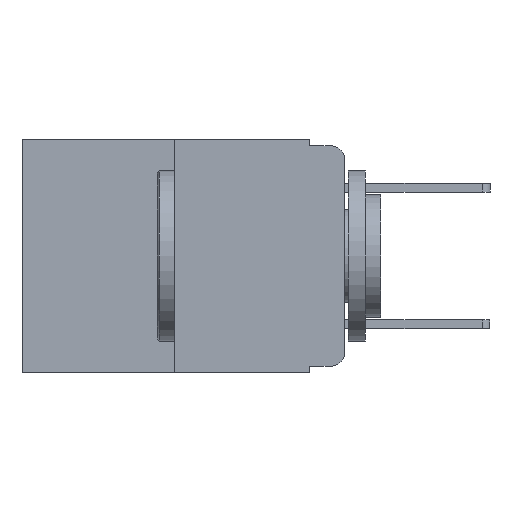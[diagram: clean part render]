
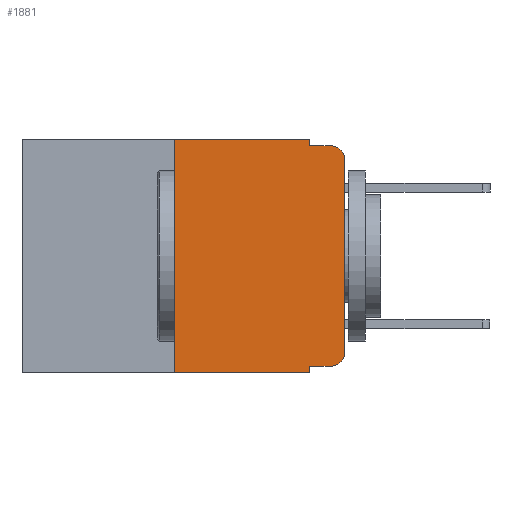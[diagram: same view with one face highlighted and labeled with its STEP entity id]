
A CAD part, left-side view. The second image highlights one B-rep face of the part: STEP entity #1881.
In plain terms, the highlighted planar face has unit normal (-1, 0, 0).
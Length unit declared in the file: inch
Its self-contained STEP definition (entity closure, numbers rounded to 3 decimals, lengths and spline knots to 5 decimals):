
#32 = VERTEX_POINT ( 'NONE', #5158 ) ;
#38 = CARTESIAN_POINT ( 'NONE',  ( 0., 0., -0.03 ) ) ;
#203 = EDGE_CURVE ( 'NONE', #1084, #32, #5326, .T. ) ;
#222 = ORIENTED_EDGE ( 'NONE', *, *, #20302, .T. ) ;
#477 = VECTOR ( 'NONE', #18074, 39.37008 ) ;
#578 = EDGE_CURVE ( 'NONE', #7838, #6584, #17220, .T. ) ;
#1083 = VERTEX_POINT ( 'NONE', #1965 ) ;
#1084 = VERTEX_POINT ( 'NONE', #23233 ) ;
#1786 = ORIENTED_EDGE ( 'NONE', *, *, #15106, .F. ) ;
#1881 = ADVANCED_FACE ( 'NONE', ( #24767 ), #8391, .F. ) ;
#1965 = CARTESIAN_POINT ( 'NONE',  ( 0., 0.051, -0.333 ) ) ;
#3151 = DIRECTION ( 'NONE',  ( -1., 0., 0. ) ) ;
#3761 = VERTEX_POINT ( 'NONE', #13410 ) ;
#3836 = CARTESIAN_POINT ( 'NONE',  ( 0., 0.051, 0. ) ) ;
#3948 = EDGE_CURVE ( 'NONE', #3761, #16313, #25304, .T. ) ;
#3993 = ORIENTED_EDGE ( 'NONE', *, *, #7341, .F. ) ;
#4042 = VECTOR ( 'NONE', #17843, 39.37008 ) ;
#4272 = CIRCLE ( 'NONE', #21971, 0.02 ) ;
#4856 = VECTOR ( 'NONE', #9632, 39.37008 ) ;
#4881 = ORIENTED_EDGE ( 'NONE', *, *, #10734, .T. ) ;
#4943 = DIRECTION ( 'NONE',  ( 0., 0., 1. ) ) ;
#5158 = CARTESIAN_POINT ( 'NONE',  ( 0., 0.051, 0. ) ) ;
#5326 = LINE ( 'NONE', #5982, #25729 ) ;
#5420 = EDGE_CURVE ( 'NONE', #16352, #24454, #21379, .T. ) ;
#5564 = ORIENTED_EDGE ( 'NONE', *, *, #3948, .T. ) ;
#5982 = CARTESIAN_POINT ( 'NONE',  ( 0., 0.473, 0. ) ) ;
#6281 = VECTOR ( 'NONE', #4943, 39.37008 ) ;
#6502 = EDGE_CURVE ( 'NONE', #32, #7838, #22802, .T. ) ;
#6584 = VERTEX_POINT ( 'NONE', #23569 ) ;
#7341 = EDGE_CURVE ( 'NONE', #1083, #16313, #19396, .T. ) ;
#7838 = VERTEX_POINT ( 'NONE', #24963 ) ;
#8124 = DIRECTION ( 'NONE',  ( 0., -1., 0. ) ) ;
#8391 = PLANE ( 'NONE',  #11916 ) ;
#8886 = CARTESIAN_POINT ( 'NONE',  ( 0., 0., 0. ) ) ;
#9097 = CARTESIAN_POINT ( 'NONE',  ( 0., 0.473, 0. ) ) ;
#9177 = DIRECTION ( 'NONE',  ( 1., 0., 0. ) ) ;
#9498 = CARTESIAN_POINT ( 'NONE',  ( 0., 0.051, 0. ) ) ;
#9632 = DIRECTION ( 'NONE',  ( 0., -1., 0. ) ) ;
#10734 = EDGE_CURVE ( 'NONE', #24454, #6584, #20980, .T. ) ;
#10807 = VECTOR ( 'NONE', #13943, 39.37008 ) ;
#10995 = CARTESIAN_POINT ( 'NONE',  ( 0., 0.02, -0.313 ) ) ;
#11696 = LINE ( 'NONE', #18957, #6281 ) ;
#11853 = LINE ( 'NONE', #17999, #477 ) ;
#11916 = AXIS2_PLACEMENT_3D ( 'NONE', #9097, #9177, #13245 ) ;
#11947 = VECTOR ( 'NONE', #8124, 39.37008 ) ;
#12475 = ORIENTED_EDGE ( 'NONE', *, *, #203, .F. ) ;
#12910 = CARTESIAN_POINT ( 'NONE',  ( 0., 0., -0.313 ) ) ;
#13019 = DIRECTION ( 'NONE',  ( 0., 0., -1. ) ) ;
#13245 = DIRECTION ( 'NONE',  ( 0., 0., -1. ) ) ;
#13410 = CARTESIAN_POINT ( 'NONE',  ( 0., 0.25, -0.343 ) ) ;
#13437 = CARTESIAN_POINT ( 'NONE',  ( 0., 0.473, -0.343 ) ) ;
#13943 = DIRECTION ( 'NONE',  ( 0., 0., 1. ) ) ;
#14121 = DIRECTION ( 'NONE',  ( 0., -1., 0. ) ) ;
#15106 = EDGE_CURVE ( 'NONE', #3761, #1084, #11696, .T. ) ;
#15167 = CARTESIAN_POINT ( 'NONE',  ( 0., 0.02, -0.03 ) ) ;
#15232 = AXIS2_PLACEMENT_3D ( 'NONE', #15167, #3151, #17163 ) ;
#15510 = DIRECTION ( 'NONE',  ( 0., 0., -1. ) ) ;
#16313 = VERTEX_POINT ( 'NONE', #24559 ) ;
#16352 = VERTEX_POINT ( 'NONE', #12910 ) ;
#17163 = DIRECTION ( 'NONE',  ( 0., 0., -1. ) ) ;
#17220 = LINE ( 'NONE', #25060, #11947 ) ;
#17581 = VECTOR ( 'NONE', #15510, 39.37008 ) ;
#17843 = DIRECTION ( 'NONE',  ( 0., 0., -1. ) ) ;
#17999 = CARTESIAN_POINT ( 'NONE',  ( 0., 0.051, -0.333 ) ) ;
#18074 = DIRECTION ( 'NONE',  ( 0., -1., 0. ) ) ;
#18192 = VERTEX_POINT ( 'NONE', #20888 ) ;
#18957 = CARTESIAN_POINT ( 'NONE',  ( 0., 0.25, 0. ) ) ;
#19396 = LINE ( 'NONE', #3836, #4042 ) ;
#20194 = EDGE_LOOP ( 'NONE', ( #25609, #4881, #23271, #24431, #12475, #1786, #5564, #3993, #20554, #222 ) ) ;
#20302 = EDGE_CURVE ( 'NONE', #18192, #16352, #4272, .T. ) ;
#20554 = ORIENTED_EDGE ( 'NONE', *, *, #23187, .T. ) ;
#20888 = CARTESIAN_POINT ( 'NONE',  ( 0., 0.02, -0.333 ) ) ;
#20980 = CIRCLE ( 'NONE', #15232, 0.02 ) ;
#21379 = LINE ( 'NONE', #8886, #10807 ) ;
#21971 = AXIS2_PLACEMENT_3D ( 'NONE', #10995, #24761, #13019 ) ;
#22802 = LINE ( 'NONE', #9498, #17581 ) ;
#23187 = EDGE_CURVE ( 'NONE', #1083, #18192, #11853, .T. ) ;
#23233 = CARTESIAN_POINT ( 'NONE',  ( 0., 0.25, 0. ) ) ;
#23271 = ORIENTED_EDGE ( 'NONE', *, *, #578, .F. ) ;
#23569 = CARTESIAN_POINT ( 'NONE',  ( 0., 0.02, -0.01 ) ) ;
#24431 = ORIENTED_EDGE ( 'NONE', *, *, #6502, .F. ) ;
#24454 = VERTEX_POINT ( 'NONE', #38 ) ;
#24559 = CARTESIAN_POINT ( 'NONE',  ( 0., 0.051, -0.343 ) ) ;
#24761 = DIRECTION ( 'NONE',  ( -1., 0., 0. ) ) ;
#24767 = FACE_OUTER_BOUND ( 'NONE', #20194, .T. ) ;
#24963 = CARTESIAN_POINT ( 'NONE',  ( 0., 0.051, -0.01 ) ) ;
#25060 = CARTESIAN_POINT ( 'NONE',  ( 0., 0.051, -0.01 ) ) ;
#25304 = LINE ( 'NONE', #13437, #4856 ) ;
#25609 = ORIENTED_EDGE ( 'NONE', *, *, #5420, .T. ) ;
#25729 = VECTOR ( 'NONE', #14121, 39.37008 ) ;
